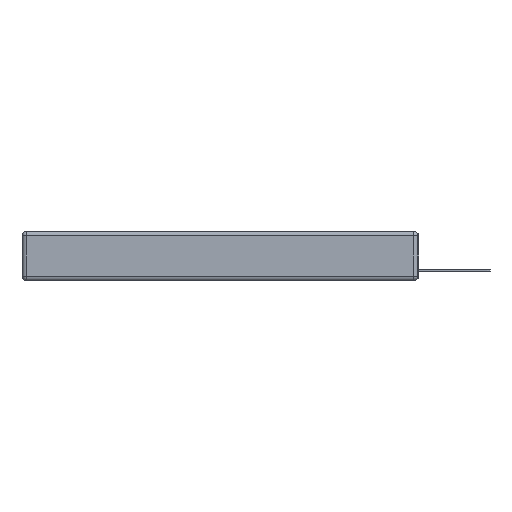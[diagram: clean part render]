
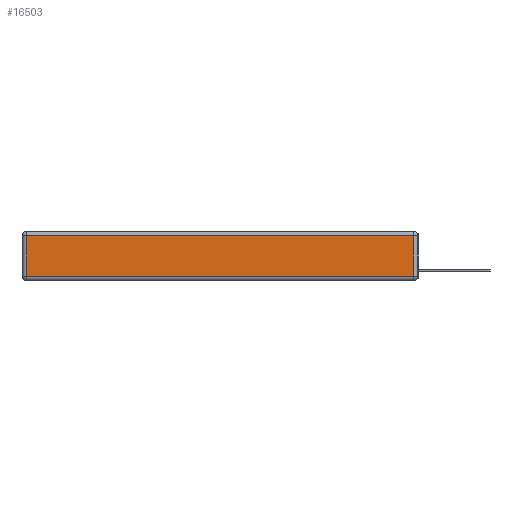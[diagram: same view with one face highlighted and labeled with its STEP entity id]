
A CAD part, left-side view. The second image highlights one B-rep face of the part: STEP entity #16503.
In plain terms, the highlighted planar face has unit normal (-1, 0, 0).
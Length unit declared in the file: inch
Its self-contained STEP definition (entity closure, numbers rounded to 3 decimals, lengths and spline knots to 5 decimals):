
#766 = ORIENTED_EDGE ( 'NONE', *, *, #5613, .T. ) ;
#2710 = VERTEX_POINT ( 'NONE', #20369 ) ;
#2913 = VERTEX_POINT ( 'NONE', #8220 ) ;
#3576 = DIRECTION ( 'NONE',  ( -1., 0., 0. ) ) ;
#4577 = CARTESIAN_POINT ( 'NONE',  ( 0., 0.03, -0.313 ) ) ;
#5503 = VERTEX_POINT ( 'NONE', #4577 ) ;
#5613 = EDGE_CURVE ( 'NONE', #2913, #5503, #10445, .T. ) ;
#6229 = VERTEX_POINT ( 'NONE', #20982 ) ;
#6604 = DIRECTION ( 'NONE',  ( 0., -1., 0. ) ) ;
#6890 = CARTESIAN_POINT ( 'NONE',  ( 0., 2.72, -0.343 ) ) ;
#7007 = VECTOR ( 'NONE', #10045, 39.37008 ) ;
#7808 = CARTESIAN_POINT ( 'NONE',  ( 0., 0.03, -0.343 ) ) ;
#8220 = CARTESIAN_POINT ( 'NONE',  ( 0., 2.72, -0.313 ) ) ;
#8312 = CARTESIAN_POINT ( 'NONE',  ( 0., 0., -0.313 ) ) ;
#8791 = EDGE_CURVE ( 'NONE', #5503, #2710, #20399, .T. ) ;
#8938 = EDGE_LOOP ( 'NONE', ( #766, #10668, #11467, #20570 ) ) ;
#9075 = LINE ( 'NONE', #6890, #7007 ) ;
#9627 = DIRECTION ( 'NONE',  ( 0., 1., 0. ) ) ;
#10025 = PLANE ( 'NONE',  #13059 ) ;
#10045 = DIRECTION ( 'NONE',  ( 0., 0., -1. ) ) ;
#10173 = EDGE_CURVE ( 'NONE', #2710, #6229, #21134, .T. ) ;
#10445 = LINE ( 'NONE', #8312, #15357 ) ;
#10668 = ORIENTED_EDGE ( 'NONE', *, *, #8791, .T. ) ;
#11467 = ORIENTED_EDGE ( 'NONE', *, *, #10173, .T. ) ;
#13059 = AXIS2_PLACEMENT_3D ( 'NONE', #18291, #3576, #20072 ) ;
#13248 = VECTOR ( 'NONE', #19291, 39.37008 ) ;
#15232 = VECTOR ( 'NONE', #9627, 39.37008 ) ;
#15357 = VECTOR ( 'NONE', #6604, 39.37008 ) ;
#16503 = ADVANCED_FACE ( 'NONE', ( #17242 ), #10025, .T. ) ;
#17242 = FACE_OUTER_BOUND ( 'NONE', #8938, .T. ) ;
#18291 = CARTESIAN_POINT ( 'NONE',  ( 0., 0., -0.343 ) ) ;
#19291 = DIRECTION ( 'NONE',  ( 0., 0., 1. ) ) ;
#20072 = DIRECTION ( 'NONE',  ( 0., 0., 1. ) ) ;
#20369 = CARTESIAN_POINT ( 'NONE',  ( 0., 0.03, -0.03 ) ) ;
#20399 = LINE ( 'NONE', #7808, #13248 ) ;
#20570 = ORIENTED_EDGE ( 'NONE', *, *, #20824, .T. ) ;
#20824 = EDGE_CURVE ( 'NONE', #6229, #2913, #9075, .T. ) ;
#20956 = CARTESIAN_POINT ( 'NONE',  ( 0., 2.75, -0.03 ) ) ;
#20982 = CARTESIAN_POINT ( 'NONE',  ( 0., 2.72, -0.03 ) ) ;
#21134 = LINE ( 'NONE', #20956, #15232 ) ;
